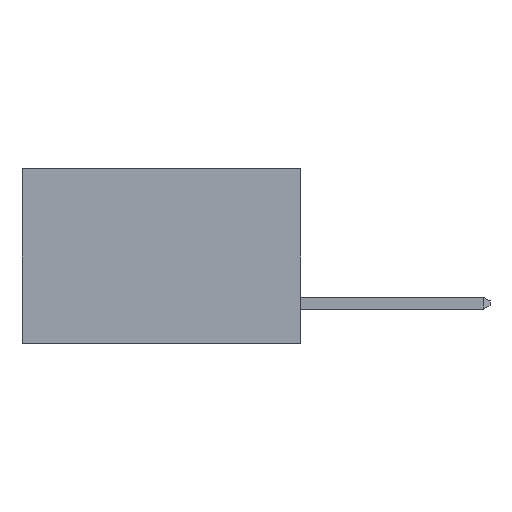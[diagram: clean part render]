
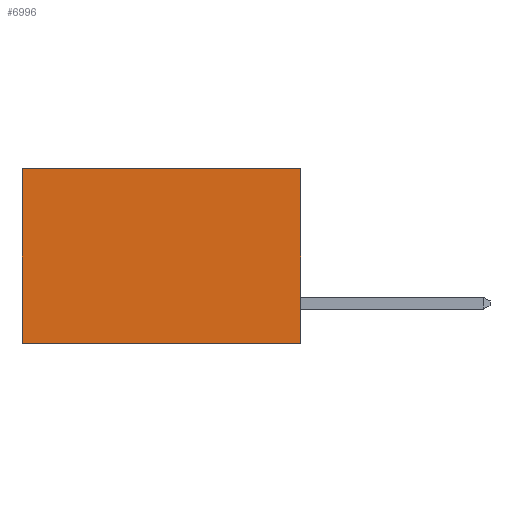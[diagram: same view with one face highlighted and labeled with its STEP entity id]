
A CAD part, left-side view. The second image highlights one B-rep face of the part: STEP entity #6996.
In plain terms, the highlighted planar face has unit normal (-1, 0, 0).
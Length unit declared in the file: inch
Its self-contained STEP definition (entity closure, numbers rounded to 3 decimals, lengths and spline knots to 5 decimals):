
#37 = DIRECTION ( 'NONE',  ( 0., 0., -1. ) ) ;
#46 = DIRECTION ( 'NONE',  ( 1., 0., 0. ) ) ;
#55 = CARTESIAN_POINT ( 'NONE',  ( 0.277, 0., -0.37 ) ) ;
#105 = AXIS2_PLACEMENT_3D ( 'NONE', #55, #46, #37 ) ;
#124 = PLANE ( 'NONE',  #105 ) ;
#1269 = CARTESIAN_POINT ( 'NONE',  ( 0.277, 0.59, -0.37 ) ) ;
#1536 = CARTESIAN_POINT ( 'NONE',  ( 0.277, 0.59, -0.37 ) ) ;
#1593 = DIRECTION ( 'NONE',  ( 0., 1., 0. ) ) ;
#2126 = EDGE_CURVE ( 'NONE', #4621, #4291, #6832, .T. ) ;
#2239 = CARTESIAN_POINT ( 'NONE',  ( 0.277, 0., -0.37 ) ) ;
#2962 = ORIENTED_EDGE ( 'NONE', *, *, #3264, .T. ) ;
#3021 = CARTESIAN_POINT ( 'NONE',  ( 0.277, 0., 0. ) ) ;
#3264 = EDGE_CURVE ( 'NONE', #5250, #4291, #3900, .T. ) ;
#3279 = ORIENTED_EDGE ( 'NONE', *, *, #2126, .F. ) ;
#3535 = DIRECTION ( 'NONE',  ( 0., 0., -1. ) ) ;
#3605 = CARTESIAN_POINT ( 'NONE',  ( 0.277, 0.59, 0. ) ) ;
#3604 = CARTESIAN_POINT ( 'NONE',  ( 0.277, 0., -0.37 ) ) ;
#3900 = LINE ( 'NONE', #1536, #5733 ) ;
#3909 = ORIENTED_EDGE ( 'NONE', *, *, #7802, .F. ) ;
#3922 = LINE ( 'NONE', #3604, #7695 ) ;
#3943 = FACE_OUTER_BOUND ( 'NONE', #5932, .T. ) ;
#4041 = ORIENTED_EDGE ( 'NONE', *, *, #7009, .T. ) ;
#4291 = VERTEX_POINT ( 'NONE', #1269 ) ;
#4415 = VERTEX_POINT ( 'NONE', #6140 ) ;
#4533 = DIRECTION ( 'NONE',  ( 0., 1., 0. ) ) ;
#4539 = DIRECTION ( 'NONE',  ( 0., 0., -1. ) ) ;
#4621 = VERTEX_POINT ( 'NONE', #8275 ) ;
#5250 = VERTEX_POINT ( 'NONE', #3605 ) ;
#5733 = VECTOR ( 'NONE', #4539, 39.37008 ) ;
#5932 = EDGE_LOOP ( 'NONE', ( #2962, #3279, #3909, #4041 ) ) ;
#6140 = CARTESIAN_POINT ( 'NONE',  ( 0.277, 0., 0. ) ) ;
#6832 = LINE ( 'NONE', #2239, #8538 ) ;
#6996 = ADVANCED_FACE ( 'NONE', ( #3943 ), #124, .F. ) ;
#7009 = EDGE_CURVE ( 'NONE', #4415, #5250, #7295, .T. ) ;
#7083 = VECTOR ( 'NONE', #1593, 39.37008 ) ;
#7295 = LINE ( 'NONE', #3021, #7083 ) ;
#7695 = VECTOR ( 'NONE', #3535, 39.37008 ) ;
#7802 = EDGE_CURVE ( 'NONE', #4415, #4621, #3922, .T. ) ;
#8275 = CARTESIAN_POINT ( 'NONE',  ( 0.277, 0., -0.37 ) ) ;
#8538 = VECTOR ( 'NONE', #4533, 39.37008 ) ;
